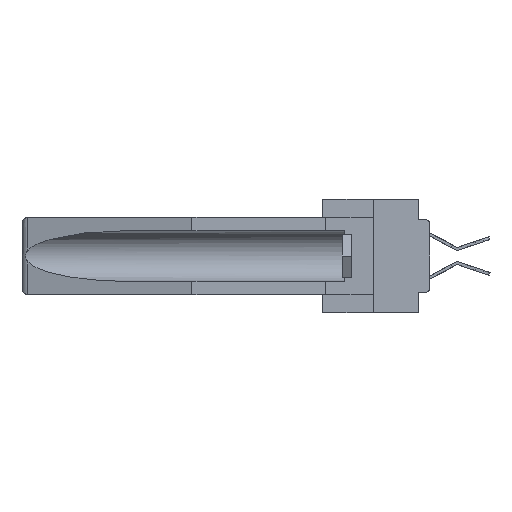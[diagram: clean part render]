
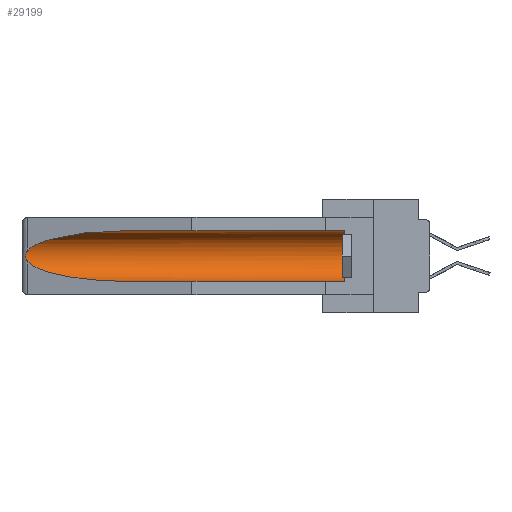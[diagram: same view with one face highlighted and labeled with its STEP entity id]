
A CAD part, left-side view. The second image highlights one B-rep face of the part: STEP entity #29199.
In plain terms, the highlighted cylindrical face has radius 2.857 mm (diameter 5.715 mm), a partial arc.
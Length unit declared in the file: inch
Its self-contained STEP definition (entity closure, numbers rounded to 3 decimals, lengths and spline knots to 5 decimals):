
#381 = CARTESIAN_POINT ( 'NONE',  ( 0.155, -0.30754, -0.284 ) ) ;
#574 = VERTEX_POINT ( 'NONE', #21913 ) ;
#1628 = CARTESIAN_POINT ( 'NONE',  ( 0.26597, 1.5296, -0.19026 ) ) ;
#1961 = CARTESIAN_POINT ( 'NONE',  ( 0.21114, 1.30732, -0.059 ) ) ;
#3616 = B_SPLINE_CURVE_WITH_KNOTS ( 'NONE', 3,
 ( #29288, #6614, #19547, #4124, #16725, #16552, #11437, #19040, #1628, #32254 ),
 .UNSPECIFIED., .F., .F.,
 ( 4, 2, 2, 2, 4 ),
 ( 0., 0.00029, 0.00058, 0.00087, 0.00117 ),
 .UNSPECIFIED. ) ;
#4124 = CARTESIAN_POINT ( 'NONE',  ( 0.2673, 1.5327, -0.16383 ) ) ;
#4369 = VERTEX_POINT ( 'NONE', #13615 ) ;
#5608 = CARTESIAN_POINT ( 'NONE',  ( 0.155, 0.126, -0.284 ) ) ;
#6270 = CARTESIAN_POINT ( 'NONE',  ( 0.26537, 1.52718, -0.14972 ) ) ;
#6305 = DIRECTION ( 'NONE',  ( 0., 1., 0. ) ) ;
#6614 = CARTESIAN_POINT ( 'NONE',  ( 0.26597, 1.52961, -0.15275 ) ) ;
#6618 = VERTEX_POINT ( 'NONE', #6270 ) ;
#8193 = CARTESIAN_POINT ( 'NONE',  ( 0.155, 0.126, -0.059 ) ) ;
#8522 = CARTESIAN_POINT ( 'NONE',  ( 0.155, -0.30754, -0.059 ) ) ;
#9447 =( BOUNDED_CURVE ( )  B_SPLINE_CURVE ( 3, ( #17689, #1961, #10243, #9608 ),
 .UNSPECIFIED., .F., .F. ) 
 B_SPLINE_CURVE_WITH_KNOTS ( ( 4, 4 ),
 ( 4.71239, 6.08839 ),
 .UNSPECIFIED. ) 
 CURVE ( )  GEOMETRIC_REPRESENTATION_ITEM ( )  RATIONAL_B_SPLINE_CURVE ( ( 1., 0.848, 0.848, 1. ) ) 
 REPRESENTATION_ITEM ( '' )  );
#9608 = CARTESIAN_POINT ( 'NONE',  ( 0.26537, 1.52718, -0.14972 ) ) ;
#10243 = CARTESIAN_POINT ( 'NONE',  ( 0.25451, 1.48313, -0.09465 ) ) ;
#10705 = ORIENTED_EDGE ( 'NONE', *, *, #24729, .T. ) ;
#11437 = CARTESIAN_POINT ( 'NONE',  ( 0.2673, 1.53269, -0.17917 ) ) ;
#11609 = ORIENTED_EDGE ( 'NONE', *, *, #13097, .T. ) ;
#11787 = CARTESIAN_POINT ( 'NONE',  ( 0.21114, 1.30732, -0.284 ) ) ;
#13067 = ORIENTED_EDGE ( 'NONE', *, *, #29358, .T. ) ;
#13097 = EDGE_CURVE ( 'NONE', #6618, #574, #3616, .T. ) ;
#13615 = CARTESIAN_POINT ( 'NONE',  ( 0.155, 1.07973, -0.284 ) ) ;
#13997 = VECTOR ( 'NONE', #30195, 39.37008 ) ;
#14674 = ORIENTED_EDGE ( 'NONE', *, *, #16301, .T. ) ;
#14692 = EDGE_LOOP ( 'NONE', ( #14674, #11609, #13067, #17591, #20841, #10705 ) ) ;
#15285 = VERTEX_POINT ( 'NONE', #24559 ) ;
#16068 = AXIS2_PLACEMENT_3D ( 'NONE', #19683, #27586, #25100 ) ;
#16164 = LINE ( 'NONE', #8522, #28611 ) ;
#16301 = EDGE_CURVE ( 'NONE', #15285, #6618, #9447, .T. ) ;
#16552 = CARTESIAN_POINT ( 'NONE',  ( 0.2675, 1.53308, -0.17534 ) ) ;
#16578 = FACE_OUTER_BOUND ( 'NONE', #14692, .T. ) ;
#16725 = CARTESIAN_POINT ( 'NONE',  ( 0.2675, 1.53308, -0.16763 ) ) ;
#16917 = CARTESIAN_POINT ( 'NONE',  ( 0.25451, 1.48313, -0.24835 ) ) ;
#17591 = ORIENTED_EDGE ( 'NONE', *, *, #20548, .F. ) ;
#17689 = CARTESIAN_POINT ( 'NONE',  ( 0.155, 1.07973, -0.059 ) ) ;
#17870 = VERTEX_POINT ( 'NONE', #5608 ) ;
#18464 = DIRECTION ( 'NONE',  ( 0., 1., 0. ) ) ;
#19040 = CARTESIAN_POINT ( 'NONE',  ( 0.26655, 1.53094, -0.18657 ) ) ;
#19401 = CARTESIAN_POINT ( 'NONE',  ( 0.155, 1.07973, -0.284 ) ) ;
#19547 = CARTESIAN_POINT ( 'NONE',  ( 0.26654, 1.53092, -0.15636 ) ) ;
#19683 = CARTESIAN_POINT ( 'NONE',  ( 0.155, 0.126, -0.1715 ) ) ;
#19870 = EDGE_CURVE ( 'NONE', #17870, #24730, #24509, .T. ) ;
#20339 = AXIS2_PLACEMENT_3D ( 'NONE', #26656, #6305, #26488 ) ;
#20548 = EDGE_CURVE ( 'NONE', #17870, #4369, #22915, .T. ) ;
#20841 = ORIENTED_EDGE ( 'NONE', *, *, #19870, .T. ) ;
#21913 = CARTESIAN_POINT ( 'NONE',  ( 0.26537, 1.52718, -0.19328 ) ) ;
#22915 = LINE ( 'NONE', #381, #13997 ) ;
#22966 =( BOUNDED_CURVE ( )  B_SPLINE_CURVE ( 3, ( #29645, #16917, #11787, #19401 ),
 .UNSPECIFIED., .F., .F. ) 
 B_SPLINE_CURVE_WITH_KNOTS ( ( 4, 4 ),
 ( 0.1948, 1.5708 ),
 .UNSPECIFIED. ) 
 CURVE ( )  GEOMETRIC_REPRESENTATION_ITEM ( )  RATIONAL_B_SPLINE_CURVE ( ( 1., 0.848, 0.848, 1. ) ) 
 REPRESENTATION_ITEM ( '' )  );
#24509 = CIRCLE ( 'NONE', #16068, 0.1125 ) ;
#24559 = CARTESIAN_POINT ( 'NONE',  ( 0.155, 1.07973, -0.059 ) ) ;
#24729 = EDGE_CURVE ( 'NONE', #24730, #15285, #16164, .T. ) ;
#24730 = VERTEX_POINT ( 'NONE', #8193 ) ;
#25100 = DIRECTION ( 'NONE',  ( 0., 0., 1. ) ) ;
#26488 = DIRECTION ( 'NONE',  ( 0., 0., 1. ) ) ;
#26656 = CARTESIAN_POINT ( 'NONE',  ( 0.155, -0.30754, -0.1715 ) ) ;
#27586 = DIRECTION ( 'NONE',  ( 0., -1., 0. ) ) ;
#28611 = VECTOR ( 'NONE', #18464, 39.37008 ) ;
#28978 = CYLINDRICAL_SURFACE ( 'NONE', #20339, 0.1125 ) ;
#29199 = ADVANCED_FACE ( 'NONE', ( #16578 ), #28978, .F. ) ;
#29288 = CARTESIAN_POINT ( 'NONE',  ( 0.26537, 1.52718, -0.14972 ) ) ;
#29358 = EDGE_CURVE ( 'NONE', #574, #4369, #22966, .T. ) ;
#29645 = CARTESIAN_POINT ( 'NONE',  ( 0.26537, 1.52718, -0.19328 ) ) ;
#30195 = DIRECTION ( 'NONE',  ( 0., 1., 0. ) ) ;
#32254 = CARTESIAN_POINT ( 'NONE',  ( 0.26537, 1.52718, -0.19328 ) ) ;
